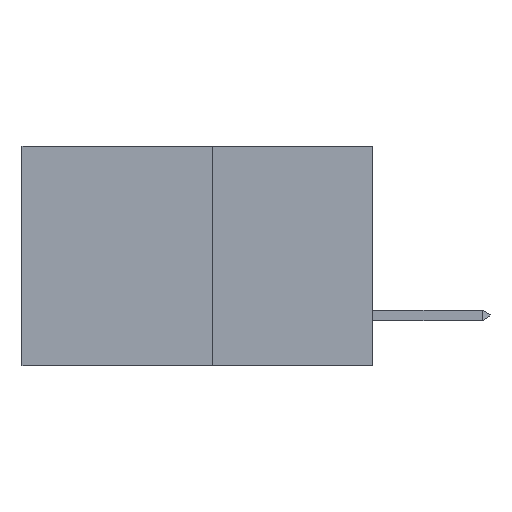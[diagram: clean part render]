
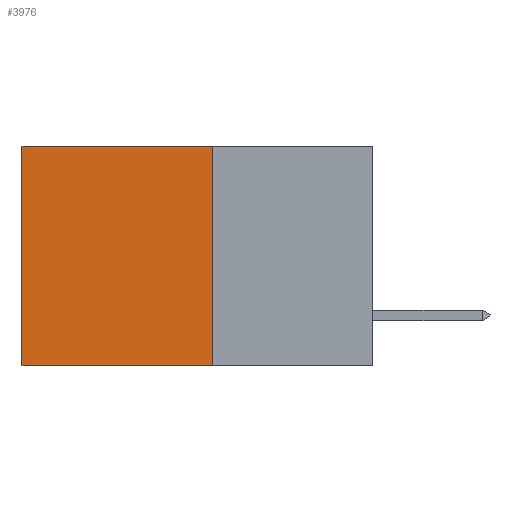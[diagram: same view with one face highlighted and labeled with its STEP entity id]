
A CAD part, left-side view. The second image highlights one B-rep face of the part: STEP entity #3976.
In plain terms, the highlighted planar face has unit normal (-1, 0, 0).
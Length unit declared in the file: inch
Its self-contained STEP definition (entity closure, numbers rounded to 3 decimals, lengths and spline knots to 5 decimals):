
#147 = VERTEX_POINT ( 'NONE', #13792 ) ;
#488 = CARTESIAN_POINT ( 'NONE',  ( 0.277, 0.27, -0.37 ) ) ;
#1853 = EDGE_LOOP ( 'NONE', ( #17073, #21620, #12637, #6252 ) ) ;
#2657 = EDGE_CURVE ( 'NONE', #15015, #25549, #8686, .T. ) ;
#2851 = VECTOR ( 'NONE', #17107, 39.37008 ) ;
#3877 = EDGE_CURVE ( 'NONE', #8022, #25549, #17865, .T. ) ;
#3976 = ADVANCED_FACE ( 'NONE', ( #8617 ), #25118, .F. ) ;
#5125 = CARTESIAN_POINT ( 'NONE',  ( 0.277, 0.59, -0.37 ) ) ;
#6252 = ORIENTED_EDGE ( 'NONE', *, *, #10084, .T. ) ;
#6703 = DIRECTION ( 'NONE',  ( 0., 0., -1. ) ) ;
#6835 = CARTESIAN_POINT ( 'NONE',  ( 0.277, 0.27, -0.37 ) ) ;
#7803 = DIRECTION ( 'NONE',  ( 1., 0., 0. ) ) ;
#7813 = AXIS2_PLACEMENT_3D ( 'NONE', #488, #7803, #6703 ) ;
#8022 = VERTEX_POINT ( 'NONE', #6835 ) ;
#8617 = FACE_OUTER_BOUND ( 'NONE', #1853, .T. ) ;
#8686 = LINE ( 'NONE', #14773, #2851 ) ;
#10084 = EDGE_CURVE ( 'NONE', #147, #15015, #27911, .T. ) ;
#12031 = DIRECTION ( 'NONE',  ( 0., 1., 0. ) ) ;
#12087 = VECTOR ( 'NONE', #12031, 39.37008 ) ;
#12637 = ORIENTED_EDGE ( 'NONE', *, *, #12864, .F. ) ;
#12864 = EDGE_CURVE ( 'NONE', #147, #8022, #21079, .T. ) ;
#13792 = CARTESIAN_POINT ( 'NONE',  ( 0.277, 0.27, 0. ) ) ;
#14773 = CARTESIAN_POINT ( 'NONE',  ( 0.277, 0.59, -0.37 ) ) ;
#15015 = VERTEX_POINT ( 'NONE', #24035 ) ;
#17073 = ORIENTED_EDGE ( 'NONE', *, *, #2657, .T. ) ;
#17107 = DIRECTION ( 'NONE',  ( 0., 0., -1. ) ) ;
#17196 = VECTOR ( 'NONE', #20830, 39.37008 ) ;
#17865 = LINE ( 'NONE', #25334, #17196 ) ;
#18707 = CARTESIAN_POINT ( 'NONE',  ( 0.277, 0.27, -0.37 ) ) ;
#20830 = DIRECTION ( 'NONE',  ( 0., 1., 0. ) ) ;
#21079 = LINE ( 'NONE', #18707, #26090 ) ;
#21620 = ORIENTED_EDGE ( 'NONE', *, *, #3877, .F. ) ;
#23053 = DIRECTION ( 'NONE',  ( 0., 0., -1. ) ) ;
#24035 = CARTESIAN_POINT ( 'NONE',  ( 0.277, 0.59, 0. ) ) ;
#24988 = CARTESIAN_POINT ( 'NONE',  ( 0.277, 0.27, 0. ) ) ;
#25118 = PLANE ( 'NONE',  #7813 ) ;
#25334 = CARTESIAN_POINT ( 'NONE',  ( 0.277, 0.27, -0.37 ) ) ;
#25549 = VERTEX_POINT ( 'NONE', #5125 ) ;
#26090 = VECTOR ( 'NONE', #23053, 39.37008 ) ;
#27911 = LINE ( 'NONE', #24988, #12087 ) ;
